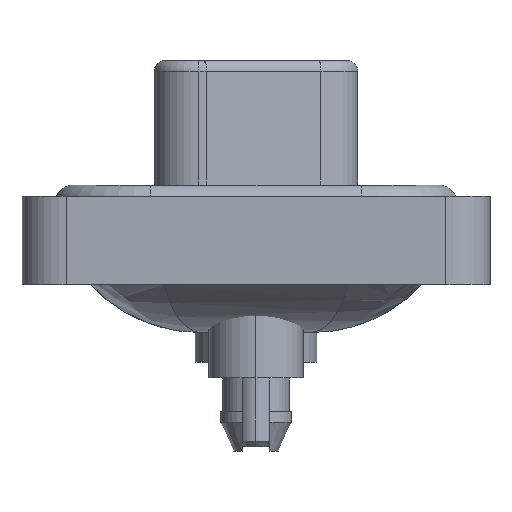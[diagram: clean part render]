
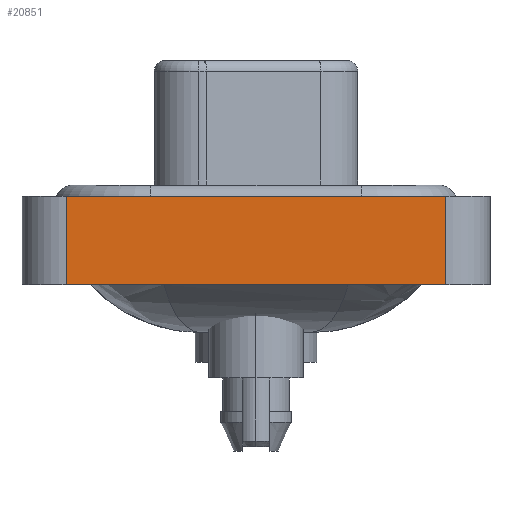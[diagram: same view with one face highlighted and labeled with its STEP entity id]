
A CAD part, left-side view. The second image highlights one B-rep face of the part: STEP entity #20851.
In plain terms, the highlighted planar face has unit normal (-1, 0, 0).
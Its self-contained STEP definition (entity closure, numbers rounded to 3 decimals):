
#66 = EDGE_CURVE ( 'NONE', #19121, #9164, #20674, .T. ) ;
#1282 = DIRECTION ( 'NONE',  ( 0., 0., 1. ) ) ;
#1568 = VERTEX_POINT ( 'NONE', #21333 ) ;
#1814 = CARTESIAN_POINT ( 'NONE',  ( -7.35, 8.55, 0.4 ) ) ;
#4041 = PLANE ( 'NONE',  #13117 ) ;
#5023 = VECTOR ( 'NONE', #15308, 1000. ) ;
#6213 = CARTESIAN_POINT ( 'NONE',  ( -7.35, -8.55, -3.6 ) ) ;
#7374 = LINE ( 'NONE', #14474, #14845 ) ;
#8257 = CARTESIAN_POINT ( 'NONE',  ( -7.35, -8.55, -3.6 ) ) ;
#9164 = VERTEX_POINT ( 'NONE', #1814 ) ;
#10108 = CARTESIAN_POINT ( 'NONE',  ( -7.35, 8.55, -3.6 ) ) ;
#10233 = LINE ( 'NONE', #8257, #15426 ) ;
#11133 = CARTESIAN_POINT ( 'NONE',  ( -7.35, -8.55, -3.6 ) ) ;
#11193 = ORIENTED_EDGE ( 'NONE', *, *, #66, .F. ) ;
#12643 = EDGE_CURVE ( 'NONE', #14112, #1568, #10233, .T. ) ;
#12768 = CARTESIAN_POINT ( 'NONE',  ( -7.35, -8.55, -3.6 ) ) ;
#12924 = EDGE_CURVE ( 'NONE', #19121, #14112, #16674, .T. ) ;
#13117 = AXIS2_PLACEMENT_3D ( 'NONE', #11133, #18199, #16474 ) ;
#14112 = VERTEX_POINT ( 'NONE', #12768 ) ;
#14474 = CARTESIAN_POINT ( 'NONE',  ( -7.35, -8.55, 0.4 ) ) ;
#14654 = EDGE_LOOP ( 'NONE', ( #18138, #16217, #11193, #21845 ) ) ;
#14845 = VECTOR ( 'NONE', #16320, 1000. ) ;
#15308 = DIRECTION ( 'NONE',  ( 0., -1., 0. ) ) ;
#15426 = VECTOR ( 'NONE', #20797, 1000. ) ;
#16217 = ORIENTED_EDGE ( 'NONE', *, *, #18163, .F. ) ;
#16320 = DIRECTION ( 'NONE',  ( 0., -1., 0. ) ) ;
#16474 = DIRECTION ( 'NONE',  ( 0., 0., 1. ) ) ;
#16674 = LINE ( 'NONE', #6213, #5023 ) ;
#17963 = CARTESIAN_POINT ( 'NONE',  ( -7.35, 8.55, -3.6 ) ) ;
#18138 = ORIENTED_EDGE ( 'NONE', *, *, #12643, .T. ) ;
#18163 = EDGE_CURVE ( 'NONE', #9164, #1568, #7374, .T. ) ;
#18199 = DIRECTION ( 'NONE',  ( -1., 0., 0. ) ) ;
#19121 = VERTEX_POINT ( 'NONE', #17963 ) ;
#19947 = FACE_OUTER_BOUND ( 'NONE', #14654, .T. ) ;
#20048 = VECTOR ( 'NONE', #1282, 1000. ) ;
#20674 = LINE ( 'NONE', #10108, #20048 ) ;
#20797 = DIRECTION ( 'NONE',  ( 0., 0., 1. ) ) ;
#20851 = ADVANCED_FACE ( 'NONE', ( #19947 ), #4041, .T. ) ;
#21333 = CARTESIAN_POINT ( 'NONE',  ( -7.35, -8.55, 0.4 ) ) ;
#21845 = ORIENTED_EDGE ( 'NONE', *, *, #12924, .T. ) ;
